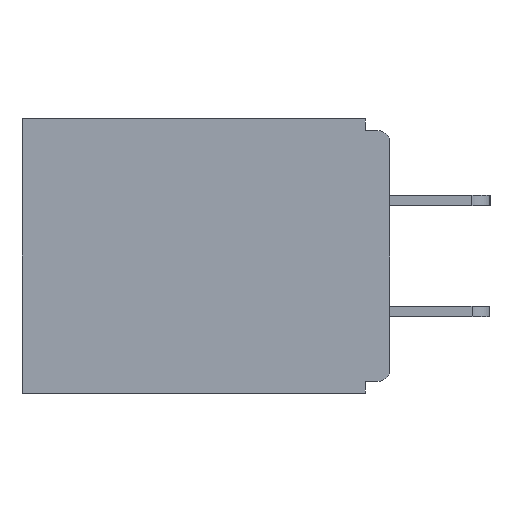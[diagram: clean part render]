
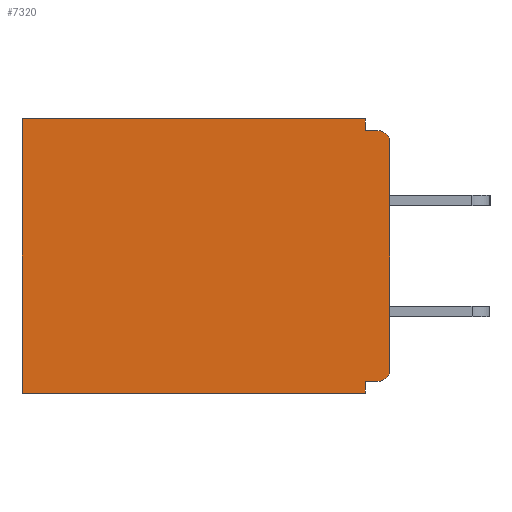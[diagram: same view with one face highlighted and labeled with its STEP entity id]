
A CAD part, left-side view. The second image highlights one B-rep face of the part: STEP entity #7320.
In plain terms, the highlighted planar face has unit normal (-1, 0, 0).
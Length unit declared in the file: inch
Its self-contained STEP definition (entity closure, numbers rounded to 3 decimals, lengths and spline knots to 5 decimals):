
#482 = VERTEX_POINT ( 'NONE', #15130 ) ;
#710 = DIRECTION ( 'NONE',  ( 0., 0., -1. ) ) ;
#1330 = VERTEX_POINT ( 'NONE', #5656 ) ;
#1670 = AXIS2_PLACEMENT_3D ( 'NONE', #8135, #16410, #16608 ) ;
#1866 = FACE_OUTER_BOUND ( 'NONE', #25793, .T. ) ;
#1946 = CARTESIAN_POINT ( 'NONE',  ( 0.298, 0.031, -0.343 ) ) ;
#1978 = LINE ( 'NONE', #13782, #15947 ) ;
#2352 = VECTOR ( 'NONE', #9456, 39.37008 ) ;
#2385 = PLANE ( 'NONE',  #6690 ) ;
#2635 = VECTOR ( 'NONE', #23906, 39.37008 ) ;
#2706 = CARTESIAN_POINT ( 'NONE',  ( 0.298, 0.031, -0.015 ) ) ;
#3135 = ORIENTED_EDGE ( 'NONE', *, *, #11441, .F. ) ;
#3358 = CARTESIAN_POINT ( 'NONE',  ( 0.298, 0.031, -0.343 ) ) ;
#4519 = AXIS2_PLACEMENT_3D ( 'NONE', #26378, #26467, #710 ) ;
#5183 = VERTEX_POINT ( 'NONE', #17799 ) ;
#5347 = DIRECTION ( 'NONE',  ( 0., 1., 0. ) ) ;
#5656 = CARTESIAN_POINT ( 'NONE',  ( 0.298, 0.015, -0.328 ) ) ;
#5767 = CARTESIAN_POINT ( 'NONE',  ( 0.298, 0., -0.313 ) ) ;
#6101 = VECTOR ( 'NONE', #5347, 39.37008 ) ;
#6542 = VERTEX_POINT ( 'NONE', #17465 ) ;
#6690 = AXIS2_PLACEMENT_3D ( 'NONE', #19952, #26244, #9099 ) ;
#6761 = EDGE_CURVE ( 'NONE', #10857, #482, #9582, .T. ) ;
#6902 = EDGE_CURVE ( 'NONE', #23403, #6542, #1978, .T. ) ;
#7306 = LINE ( 'NONE', #1946, #23051 ) ;
#7320 = ADVANCED_FACE ( 'NONE', ( #1866 ), #2385, .F. ) ;
#7420 = DIRECTION ( 'NONE',  ( 0., -1., 0. ) ) ;
#7743 = CARTESIAN_POINT ( 'NONE',  ( 0.298, 0., -0.03 ) ) ;
#8135 = CARTESIAN_POINT ( 'NONE',  ( 0.298, 0.015, -0.313 ) ) ;
#9099 = DIRECTION ( 'NONE',  ( 0., 0., -1. ) ) ;
#9456 = DIRECTION ( 'NONE',  ( 0., 0., -1. ) ) ;
#9563 = LINE ( 'NONE', #23683, #11887 ) ;
#9582 = CIRCLE ( 'NONE', #4519, 0.015 ) ;
#10587 = ORIENTED_EDGE ( 'NONE', *, *, #15425, .F. ) ;
#10857 = VERTEX_POINT ( 'NONE', #7743 ) ;
#11357 = ORIENTED_EDGE ( 'NONE', *, *, #6902, .T. ) ;
#11441 = EDGE_CURVE ( 'NONE', #23403, #19083, #7306, .T. ) ;
#11443 = ORIENTED_EDGE ( 'NONE', *, *, #19198, .T. ) ;
#11710 = EDGE_CURVE ( 'NONE', #10857, #22233, #13987, .T. ) ;
#11887 = VECTOR ( 'NONE', #13052, 39.37008 ) ;
#12052 = VERTEX_POINT ( 'NONE', #17106 ) ;
#12137 = VERTEX_POINT ( 'NONE', #13615 ) ;
#13052 = DIRECTION ( 'NONE',  ( 0., 1., 0. ) ) ;
#13181 = CARTESIAN_POINT ( 'NONE',  ( 0.298, 0., 0. ) ) ;
#13615 = CARTESIAN_POINT ( 'NONE',  ( 0.298, 0.46, -0.343 ) ) ;
#13689 = LINE ( 'NONE', #22014, #2352 ) ;
#13782 = CARTESIAN_POINT ( 'NONE',  ( 0.298, 0., 0. ) ) ;
#13987 = LINE ( 'NONE', #13181, #2635 ) ;
#15130 = CARTESIAN_POINT ( 'NONE',  ( 0.298, 0.015, -0.015 ) ) ;
#15425 = EDGE_CURVE ( 'NONE', #1330, #5183, #9563, .T. ) ;
#15466 = EDGE_CURVE ( 'NONE', #5183, #12052, #24972, .T. ) ;
#15923 = DIRECTION ( 'NONE',  ( 0., 1., 0. ) ) ;
#15947 = VECTOR ( 'NONE', #15923, 39.37008 ) ;
#16174 = ORIENTED_EDGE ( 'NONE', *, *, #19467, .T. ) ;
#16410 = DIRECTION ( 'NONE',  ( -1., 0., 0. ) ) ;
#16608 = DIRECTION ( 'NONE',  ( 0., 0., -1. ) ) ;
#17106 = CARTESIAN_POINT ( 'NONE',  ( 0.298, 0.031, -0.343 ) ) ;
#17465 = CARTESIAN_POINT ( 'NONE',  ( 0.298, 0.46, 0. ) ) ;
#17799 = CARTESIAN_POINT ( 'NONE',  ( 0.298, 0.031, -0.328 ) ) ;
#18109 = CARTESIAN_POINT ( 'NONE',  ( 0.298, 0., -0.343 ) ) ;
#18429 = LINE ( 'NONE', #18109, #6101 ) ;
#19083 = VERTEX_POINT ( 'NONE', #2706 ) ;
#19198 = EDGE_CURVE ( 'NONE', #1330, #22233, #21090, .T. ) ;
#19467 = EDGE_CURVE ( 'NONE', #6542, #12137, #13689, .T. ) ;
#19952 = CARTESIAN_POINT ( 'NONE',  ( 0.298, 0., 0. ) ) ;
#21090 = CIRCLE ( 'NONE', #1670, 0.015 ) ;
#21669 = ORIENTED_EDGE ( 'NONE', *, *, #6761, .T. ) ;
#21861 = ORIENTED_EDGE ( 'NONE', *, *, #15466, .F. ) ;
#22014 = CARTESIAN_POINT ( 'NONE',  ( 0.298, 0.46, 0. ) ) ;
#22233 = VERTEX_POINT ( 'NONE', #5767 ) ;
#22318 = ORIENTED_EDGE ( 'NONE', *, *, #24407, .F. ) ;
#22740 = ORIENTED_EDGE ( 'NONE', *, *, #24071, .F. ) ;
#22772 = CARTESIAN_POINT ( 'NONE',  ( 0.298, 0., -0.015 ) ) ;
#22860 = LINE ( 'NONE', #22772, #25856 ) ;
#23051 = VECTOR ( 'NONE', #27702, 39.37008 ) ;
#23403 = VERTEX_POINT ( 'NONE', #24767 ) ;
#23683 = CARTESIAN_POINT ( 'NONE',  ( 0.298, 0., -0.328 ) ) ;
#23906 = DIRECTION ( 'NONE',  ( 0., 0., -1. ) ) ;
#24071 = EDGE_CURVE ( 'NONE', #19083, #482, #22860, .T. ) ;
#24407 = EDGE_CURVE ( 'NONE', #12052, #12137, #18429, .T. ) ;
#24767 = CARTESIAN_POINT ( 'NONE',  ( 0.298, 0.031, 0. ) ) ;
#24972 = LINE ( 'NONE', #3358, #25336 ) ;
#25058 = ORIENTED_EDGE ( 'NONE', *, *, #11710, .F. ) ;
#25336 = VECTOR ( 'NONE', #26773, 39.37008 ) ;
#25793 = EDGE_LOOP ( 'NONE', ( #21669, #22740, #3135, #11357, #16174, #22318, #21861, #10587, #11443, #25058 ) ) ;
#25856 = VECTOR ( 'NONE', #7420, 39.37008 ) ;
#26244 = DIRECTION ( 'NONE',  ( 1., 0., 0. ) ) ;
#26378 = CARTESIAN_POINT ( 'NONE',  ( 0.298, 0.015, -0.03 ) ) ;
#26467 = DIRECTION ( 'NONE',  ( -1., 0., 0. ) ) ;
#26773 = DIRECTION ( 'NONE',  ( 0., 0., -1. ) ) ;
#27702 = DIRECTION ( 'NONE',  ( 0., 0., -1. ) ) ;
